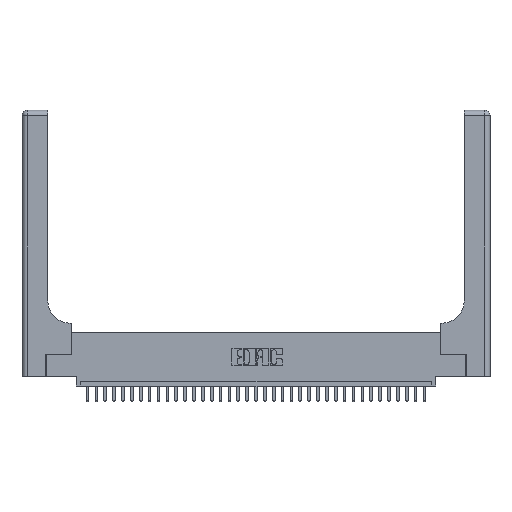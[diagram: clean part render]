
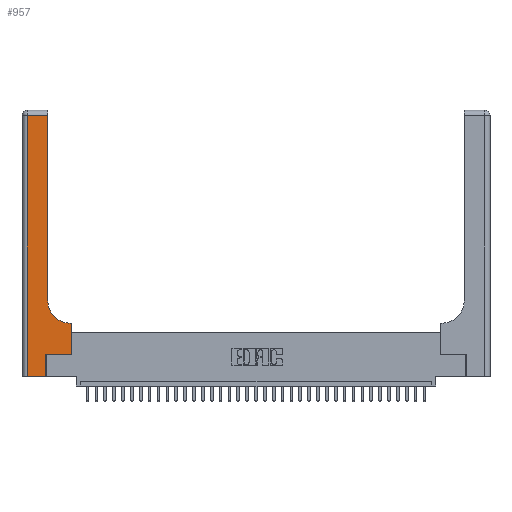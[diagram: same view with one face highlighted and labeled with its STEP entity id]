
A CAD part, top view. The second image highlights one B-rep face of the part: STEP entity #957.
In plain terms, the highlighted planar face has unit normal (0, 0, 1).
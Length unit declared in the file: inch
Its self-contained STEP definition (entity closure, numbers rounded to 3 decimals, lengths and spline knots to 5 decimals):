
#265 = EDGE_CURVE ( 'NONE', #24312, #12637, #8352, .T. ) ;
#957 = ADVANCED_FACE ( 'NONE', ( #2355 ), #29885, .F. ) ;
#1973 = CARTESIAN_POINT ( 'NONE',  ( 0.2915, 3., 0.37 ) ) ;
#2133 = VECTOR ( 'NONE', #24801, 39.37008 ) ;
#2355 = FACE_OUTER_BOUND ( 'NONE', #17180, .T. ) ;
#2952 = VECTOR ( 'NONE', #9705, 39.37008 ) ;
#4518 = EDGE_CURVE ( 'NONE', #13455, #5950, #16801, .T. ) ;
#4968 = AXIS2_PLACEMENT_3D ( 'NONE', #14339, #28402, #26512 ) ;
#5950 = VERTEX_POINT ( 'NONE', #28330 ) ;
#6218 = CARTESIAN_POINT ( 'NONE',  ( 0.269, 0.25, 0.37 ) ) ;
#6510 = LINE ( 'NONE', #1973, #34606 ) ;
#7442 = CARTESIAN_POINT ( 'NONE',  ( 0., 0., 0.37 ) ) ;
#7454 = CARTESIAN_POINT ( 'NONE',  ( 0.2915, 0.6, 0.37 ) ) ;
#8304 = DIRECTION ( 'NONE',  ( 0., 0., -1. ) ) ;
#8352 = CIRCLE ( 'NONE', #22699, 0.25 ) ;
#8419 = CARTESIAN_POINT ( 'NONE',  ( 0.5585, 0.6, 0.37 ) ) ;
#8530 = VERTEX_POINT ( 'NONE', #15539 ) ;
#8563 = CARTESIAN_POINT ( 'NONE',  ( 0., 2.94, 0.37 ) ) ;
#8754 = EDGE_CURVE ( 'NONE', #22826, #8530, #21188, .T. ) ;
#9624 = VECTOR ( 'NONE', #14600, 39.37008 ) ;
#9658 = DIRECTION ( 'NONE',  ( 0., 1., 0. ) ) ;
#9705 = DIRECTION ( 'NONE',  ( -1., 0., 0. ) ) ;
#9753 = VERTEX_POINT ( 'NONE', #22337 ) ;
#10207 = VERTEX_POINT ( 'NONE', #8419 ) ;
#10961 = VECTOR ( 'NONE', #13245, 39.37008 ) ;
#11516 = DIRECTION ( 'NONE',  ( 0., 1., 0. ) ) ;
#11947 = EDGE_CURVE ( 'NONE', #8530, #9753, #13293, .T. ) ;
#12637 = VERTEX_POINT ( 'NONE', #34741 ) ;
#12865 = EDGE_CURVE ( 'NONE', #10207, #24312, #25526, .T. ) ;
#13245 = DIRECTION ( 'NONE',  ( 1., 0., 0. ) ) ;
#13262 = ORIENTED_EDGE ( 'NONE', *, *, #19137, .T. ) ;
#13293 = LINE ( 'NONE', #20445, #16661 ) ;
#13455 = VERTEX_POINT ( 'NONE', #30947 ) ;
#13650 = EDGE_CURVE ( 'NONE', #5950, #22826, #16968, .T. ) ;
#14082 = CARTESIAN_POINT ( 'NONE',  ( 0.5415, 0.6, 0.37 ) ) ;
#14339 = CARTESIAN_POINT ( 'NONE',  ( 0., 3., 0.37 ) ) ;
#14578 = ORIENTED_EDGE ( 'NONE', *, *, #32266, .T. ) ;
#14600 = DIRECTION ( 'NONE',  ( -1., 0., 0. ) ) ;
#14894 = VECTOR ( 'NONE', #11516, 39.37008 ) ;
#15222 = ORIENTED_EDGE ( 'NONE', *, *, #265, .T. ) ;
#15539 = CARTESIAN_POINT ( 'NONE',  ( 0.269, 0., 0.37 ) ) ;
#16507 = ORIENTED_EDGE ( 'NONE', *, *, #4518, .T. ) ;
#16660 = CARTESIAN_POINT ( 'NONE',  ( 0.5585, 0.25, 0.37 ) ) ;
#16661 = VECTOR ( 'NONE', #9658, 39.37008 ) ;
#16801 = LINE ( 'NONE', #8563, #9624 ) ;
#16968 = LINE ( 'NONE', #24464, #2133 ) ;
#17180 = EDGE_LOOP ( 'NONE', ( #30562, #16507, #25375, #31450, #34577, #14578, #13262, #20821, #15222 ) ) ;
#18315 = LINE ( 'NONE', #27823, #14894 ) ;
#19137 = EDGE_CURVE ( 'NONE', #33831, #10207, #18315, .T. ) ;
#19281 = DIRECTION ( 'NONE',  ( 1., 0., 0. ) ) ;
#19979 = VECTOR ( 'NONE', #19281, 39.37008 ) ;
#20445 = CARTESIAN_POINT ( 'NONE',  ( 0.269, 0., 0.37 ) ) ;
#20821 = ORIENTED_EDGE ( 'NONE', *, *, #12865, .T. ) ;
#21188 = LINE ( 'NONE', #7442, #10961 ) ;
#22337 = CARTESIAN_POINT ( 'NONE',  ( 0.269, 0.25, 0.37 ) ) ;
#22699 = AXIS2_PLACEMENT_3D ( 'NONE', #30142, #8304, #32887 ) ;
#22826 = VERTEX_POINT ( 'NONE', #25347 ) ;
#24312 = VERTEX_POINT ( 'NONE', #14082 ) ;
#24464 = CARTESIAN_POINT ( 'NONE',  ( 0.06, 3., 0.37 ) ) ;
#24801 = DIRECTION ( 'NONE',  ( 0., -1., 0. ) ) ;
#25145 = EDGE_CURVE ( 'NONE', #12637, #13455, #6510, .T. ) ;
#25347 = CARTESIAN_POINT ( 'NONE',  ( 0.06, 0., 0.37 ) ) ;
#25375 = ORIENTED_EDGE ( 'NONE', *, *, #13650, .T. ) ;
#25526 = LINE ( 'NONE', #7454, #2952 ) ;
#26512 = DIRECTION ( 'NONE',  ( -1., 0., 0. ) ) ;
#27823 = CARTESIAN_POINT ( 'NONE',  ( 0.5585, 0.25, 0.37 ) ) ;
#28330 = CARTESIAN_POINT ( 'NONE',  ( 0.06, 2.94, 0.37 ) ) ;
#28402 = DIRECTION ( 'NONE',  ( 0., 0., -1. ) ) ;
#29885 = PLANE ( 'NONE',  #4968 ) ;
#30142 = CARTESIAN_POINT ( 'NONE',  ( 0.5415, 0.85, 0.37 ) ) ;
#30562 = ORIENTED_EDGE ( 'NONE', *, *, #25145, .T. ) ;
#30947 = CARTESIAN_POINT ( 'NONE',  ( 0.2915, 2.94, 0.37 ) ) ;
#31450 = ORIENTED_EDGE ( 'NONE', *, *, #8754, .T. ) ;
#31933 = LINE ( 'NONE', #6218, #19979 ) ;
#32266 = EDGE_CURVE ( 'NONE', #9753, #33831, #31933, .T. ) ;
#32887 = DIRECTION ( 'NONE',  ( 1., 0., 0. ) ) ;
#33831 = VERTEX_POINT ( 'NONE', #16660 ) ;
#34287 = DIRECTION ( 'NONE',  ( 0., 1., 0. ) ) ;
#34577 = ORIENTED_EDGE ( 'NONE', *, *, #11947, .T. ) ;
#34606 = VECTOR ( 'NONE', #34287, 39.37008 ) ;
#34741 = CARTESIAN_POINT ( 'NONE',  ( 0.2915, 0.85, 0.37 ) ) ;
